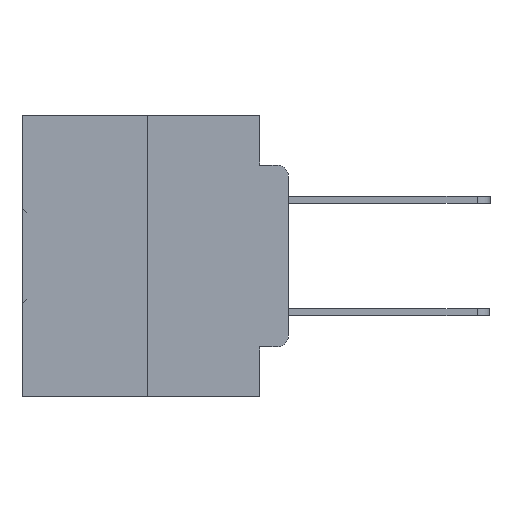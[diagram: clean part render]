
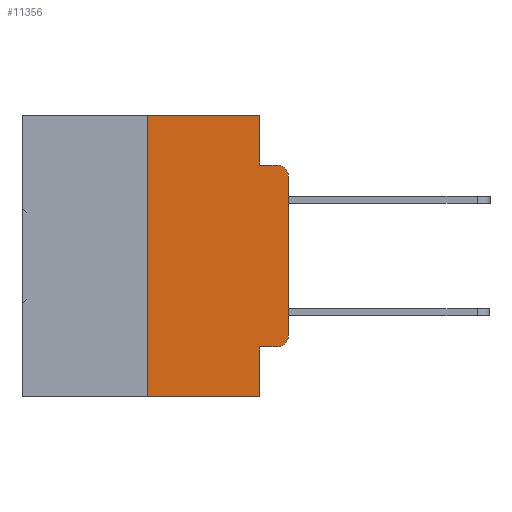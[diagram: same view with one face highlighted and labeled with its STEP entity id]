
A CAD part, left-side view. The second image highlights one B-rep face of the part: STEP entity #11356.
In plain terms, the highlighted planar face has unit normal (-1, 0, 0).
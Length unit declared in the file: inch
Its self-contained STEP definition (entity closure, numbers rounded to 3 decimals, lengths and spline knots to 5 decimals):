
#286 = EDGE_CURVE ( 'NONE', #33960, #1989, #9709, .T. ) ;
#346 = LINE ( 'NONE', #32868, #20246 ) ;
#851 = DIRECTION ( 'NONE',  ( 0., 0., -1. ) ) ;
#1087 = AXIS2_PLACEMENT_3D ( 'NONE', #5192, #24082, #7923 ) ;
#1100 = EDGE_CURVE ( 'NONE', #8108, #29902, #27269, .T. ) ;
#1147 = DIRECTION ( 'NONE',  ( 0., 0., -1. ) ) ;
#1708 = ORIENTED_EDGE ( 'NONE', *, *, #8159, .T. ) ;
#1979 = DIRECTION ( 'NONE',  ( 0., -1., 0. ) ) ;
#1989 = VERTEX_POINT ( 'NONE', #33471 ) ;
#2020 = LINE ( 'NONE', #13280, #30537 ) ;
#2320 = LINE ( 'NONE', #23057, #30042 ) ;
#2536 = EDGE_CURVE ( 'NONE', #1989, #21403, #2320, .T. ) ;
#3885 = CARTESIAN_POINT ( 'NONE',  ( 0., 0.051, 0. ) ) ;
#4093 = ORIENTED_EDGE ( 'NONE', *, *, #20910, .F. ) ;
#4787 = VERTEX_POINT ( 'NONE', #5560 ) ;
#5028 = ORIENTED_EDGE ( 'NONE', *, *, #6833, .F. ) ;
#5192 = CARTESIAN_POINT ( 'NONE',  ( 0., 0.02, -0.1085 ) ) ;
#5560 = CARTESIAN_POINT ( 'NONE',  ( 0., 0.051, 0. ) ) ;
#5734 = DIRECTION ( 'NONE',  ( -1., 0., 0. ) ) ;
#5755 = CARTESIAN_POINT ( 'NONE',  ( 0., 0.25, 0. ) ) ;
#6506 = VECTOR ( 'NONE', #1979, 39.37008 ) ;
#6833 = EDGE_CURVE ( 'NONE', #28668, #28610, #18401, .T. ) ;
#6989 = CARTESIAN_POINT ( 'NONE',  ( 0., 0.25, -0.5 ) ) ;
#7577 = ORIENTED_EDGE ( 'NONE', *, *, #21336, .F. ) ;
#7788 = DIRECTION ( 'NONE',  ( 0., 0., -1. ) ) ;
#7923 = DIRECTION ( 'NONE',  ( 0., 0., -1. ) ) ;
#8108 = VERTEX_POINT ( 'NONE', #6989 ) ;
#8159 = EDGE_CURVE ( 'NONE', #21403, #28610, #12819, .T. ) ;
#8490 = DIRECTION ( 'NONE',  ( 0., 0., 1. ) ) ;
#8727 = CARTESIAN_POINT ( 'NONE',  ( 0., 0., -0.1085 ) ) ;
#9579 = EDGE_LOOP ( 'NONE', ( #10185, #1708, #5028, #20660, #29819, #7577, #11329, #4093, #29676, #13010 ) ) ;
#9709 = CIRCLE ( 'NONE', #16321, 0.02 ) ;
#10185 = ORIENTED_EDGE ( 'NONE', *, *, #2536, .T. ) ;
#10425 = EDGE_CURVE ( 'NONE', #4787, #28668, #11845, .T. ) ;
#10979 = VECTOR ( 'NONE', #1147, 39.37008 ) ;
#11329 = ORIENTED_EDGE ( 'NONE', *, *, #1100, .T. ) ;
#11334 = DIRECTION ( 'NONE',  ( 0., -1., 0. ) ) ;
#11356 = ADVANCED_FACE ( 'NONE', ( #16427 ), #21290, .F. ) ;
#11359 = EDGE_CURVE ( 'NONE', #31492, #4787, #2020, .T. ) ;
#11636 = DIRECTION ( 'NONE',  ( 0., -1., 0. ) ) ;
#11845 = LINE ( 'NONE', #3885, #10979 ) ;
#12819 = CIRCLE ( 'NONE', #1087, 0.02 ) ;
#13010 = ORIENTED_EDGE ( 'NONE', *, *, #286, .T. ) ;
#13167 = CARTESIAN_POINT ( 'NONE',  ( 0., 0.473, 0. ) ) ;
#13280 = CARTESIAN_POINT ( 'NONE',  ( 0., 0.473, 0. ) ) ;
#13538 = CARTESIAN_POINT ( 'NONE',  ( 0., 0.051, -0.5 ) ) ;
#14323 = AXIS2_PLACEMENT_3D ( 'NONE', #13167, #23952, #7788 ) ;
#14709 = LINE ( 'NONE', #5755, #21041 ) ;
#14775 = CARTESIAN_POINT ( 'NONE',  ( 0., 0.25, 0. ) ) ;
#16321 = AXIS2_PLACEMENT_3D ( 'NONE', #29142, #5734, #26950 ) ;
#16427 = FACE_OUTER_BOUND ( 'NONE', #9579, .T. ) ;
#18401 = LINE ( 'NONE', #18626, #6506 ) ;
#18626 = CARTESIAN_POINT ( 'NONE',  ( 0., 0.051, -0.0885 ) ) ;
#19386 = CARTESIAN_POINT ( 'NONE',  ( 0., 0.051, -0.4115 ) ) ;
#19811 = VERTEX_POINT ( 'NONE', #28402 ) ;
#20246 = VECTOR ( 'NONE', #851, 39.37008 ) ;
#20392 = DIRECTION ( 'NONE',  ( 0., 0., 1. ) ) ;
#20660 = ORIENTED_EDGE ( 'NONE', *, *, #10425, .F. ) ;
#20910 = EDGE_CURVE ( 'NONE', #19811, #29902, #346, .T. ) ;
#21041 = VECTOR ( 'NONE', #8490, 39.37008 ) ;
#21289 = VECTOR ( 'NONE', #11334, 39.37008 ) ;
#21290 = PLANE ( 'NONE',  #14323 ) ;
#21336 = EDGE_CURVE ( 'NONE', #8108, #31492, #14709, .T. ) ;
#21403 = VERTEX_POINT ( 'NONE', #8727 ) ;
#23057 = CARTESIAN_POINT ( 'NONE',  ( 0., 0., 0. ) ) ;
#23482 = CARTESIAN_POINT ( 'NONE',  ( 0., 0.473, -0.5 ) ) ;
#23952 = DIRECTION ( 'NONE',  ( 1., 0., 0. ) ) ;
#24082 = DIRECTION ( 'NONE',  ( -1., 0., 0. ) ) ;
#26943 = CARTESIAN_POINT ( 'NONE',  ( 0., 0.02, -0.0885 ) ) ;
#26950 = DIRECTION ( 'NONE',  ( 0., 0., -1. ) ) ;
#27269 = LINE ( 'NONE', #23482, #32546 ) ;
#27975 = EDGE_CURVE ( 'NONE', #19811, #33960, #29155, .T. ) ;
#28402 = CARTESIAN_POINT ( 'NONE',  ( 0., 0.051, -0.4115 ) ) ;
#28610 = VERTEX_POINT ( 'NONE', #26943 ) ;
#28668 = VERTEX_POINT ( 'NONE', #32287 ) ;
#29142 = CARTESIAN_POINT ( 'NONE',  ( 0., 0.02, -0.3915 ) ) ;
#29155 = LINE ( 'NONE', #19386, #21289 ) ;
#29676 = ORIENTED_EDGE ( 'NONE', *, *, #27975, .T. ) ;
#29819 = ORIENTED_EDGE ( 'NONE', *, *, #11359, .F. ) ;
#29902 = VERTEX_POINT ( 'NONE', #13538 ) ;
#30042 = VECTOR ( 'NONE', #20392, 39.37008 ) ;
#30537 = VECTOR ( 'NONE', #31840, 39.37008 ) ;
#30896 = CARTESIAN_POINT ( 'NONE',  ( 0., 0.02, -0.4115 ) ) ;
#31492 = VERTEX_POINT ( 'NONE', #14775 ) ;
#31840 = DIRECTION ( 'NONE',  ( 0., -1., 0. ) ) ;
#32287 = CARTESIAN_POINT ( 'NONE',  ( 0., 0.051, -0.0885 ) ) ;
#32546 = VECTOR ( 'NONE', #11636, 39.37008 ) ;
#32868 = CARTESIAN_POINT ( 'NONE',  ( 0., 0.051, 0. ) ) ;
#33471 = CARTESIAN_POINT ( 'NONE',  ( 0., 0., -0.3915 ) ) ;
#33960 = VERTEX_POINT ( 'NONE', #30896 ) ;
